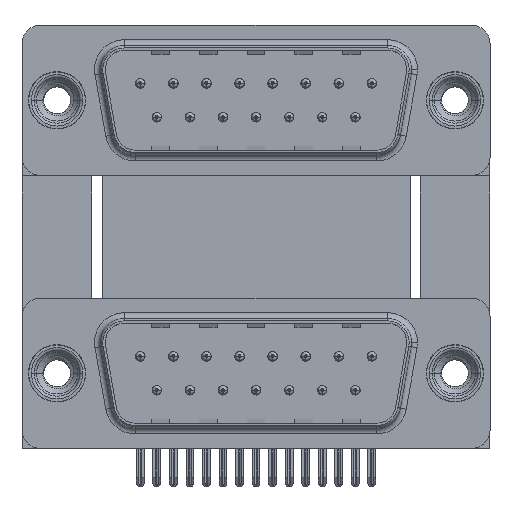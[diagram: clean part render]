
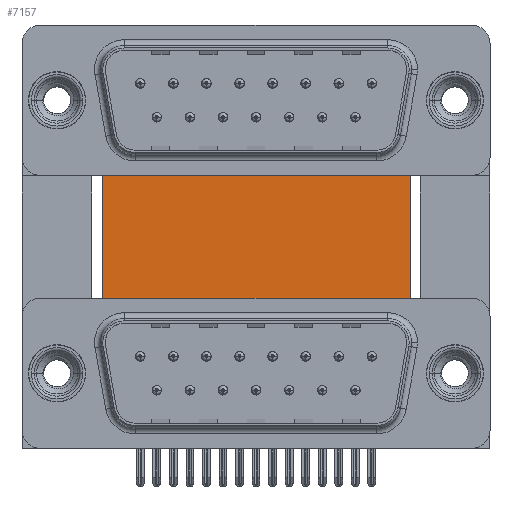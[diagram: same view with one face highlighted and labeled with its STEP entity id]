
A CAD part, top view. The second image highlights one B-rep face of the part: STEP entity #7157.
In plain terms, the highlighted planar face has unit normal (0, 0, 1).
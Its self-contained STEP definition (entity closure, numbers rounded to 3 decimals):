
#67 = LINE ( 'NONE', #24324, #22918 ) ;
#2716 = EDGE_LOOP ( 'NONE', ( #10494, #2907, #17678, #2723 ) ) ;
#2723 = ORIENTED_EDGE ( 'NONE', *, *, #3423, .T. ) ;
#2907 = ORIENTED_EDGE ( 'NONE', *, *, #10132, .F. ) ;
#2934 = CARTESIAN_POINT ( 'NONE',  ( 29.58, 16.585, -12. ) ) ;
#3423 = EDGE_CURVE ( 'NONE', #16822, #15282, #23385, .T. ) ;
#3494 = DIRECTION ( 'NONE',  ( 1., 0., 0. ) ) ;
#3684 = CARTESIAN_POINT ( 'NONE',  ( 29.58, 16.585, -12. ) ) ;
#4390 = EDGE_CURVE ( 'NONE', #16822, #25252, #67, .T. ) ;
#4975 = DIRECTION ( 'NONE',  ( 0., 0., -1. ) ) ;
#7157 = ADVANCED_FACE ( 'NONE', ( #29371 ), #19182, .F. ) ;
#7666 = DIRECTION ( 'NONE',  ( -1., 0., 0. ) ) ;
#10132 = EDGE_CURVE ( 'NONE', #25252, #29429, #15287, .T. ) ;
#10494 = ORIENTED_EDGE ( 'NONE', *, *, #13992, .T. ) ;
#11212 = DIRECTION ( 'NONE',  ( 0., -1., 0. ) ) ;
#11363 = CARTESIAN_POINT ( 'NONE',  ( 3.79, 16.585, -12. ) ) ;
#12092 = CARTESIAN_POINT ( 'NONE',  ( 3.79, 16.585, -12. ) ) ;
#13158 = LINE ( 'NONE', #27127, #17642 ) ;
#13992 = EDGE_CURVE ( 'NONE', #15282, #29429, #13158, .T. ) ;
#14542 = VECTOR ( 'NONE', #20000, 1000. ) ;
#15282 = VERTEX_POINT ( 'NONE', #20580 ) ;
#15287 = LINE ( 'NONE', #2934, #14542 ) ;
#16670 = VECTOR ( 'NONE', #11212, 1000. ) ;
#16822 = VERTEX_POINT ( 'NONE', #28156 ) ;
#17642 = VECTOR ( 'NONE', #3494, 1000. ) ;
#17678 = ORIENTED_EDGE ( 'NONE', *, *, #4390, .F. ) ;
#19182 = PLANE ( 'NONE',  #22985 ) ;
#20000 = DIRECTION ( 'NONE',  ( 0., -1., 0. ) ) ;
#20580 = CARTESIAN_POINT ( 'NONE',  ( 3.79, -3.735, -12. ) ) ;
#22918 = VECTOR ( 'NONE', #24167, 1000. ) ;
#22985 = AXIS2_PLACEMENT_3D ( 'NONE', #12092, #4975, #7666 ) ;
#23385 = LINE ( 'NONE', #11363, #16670 ) ;
#24167 = DIRECTION ( 'NONE',  ( 1., 0., 0. ) ) ;
#24324 = CARTESIAN_POINT ( 'NONE',  ( 3.79, 16.585, -12. ) ) ;
#25252 = VERTEX_POINT ( 'NONE', #3684 ) ;
#27127 = CARTESIAN_POINT ( 'NONE',  ( 3.79, -3.735, -12. ) ) ;
#28156 = CARTESIAN_POINT ( 'NONE',  ( 3.79, 16.585, -12. ) ) ;
#29371 = FACE_OUTER_BOUND ( 'NONE', #2716, .T. ) ;
#29429 = VERTEX_POINT ( 'NONE', #30282 ) ;
#30282 = CARTESIAN_POINT ( 'NONE',  ( 29.58, -3.735, -12. ) ) ;
